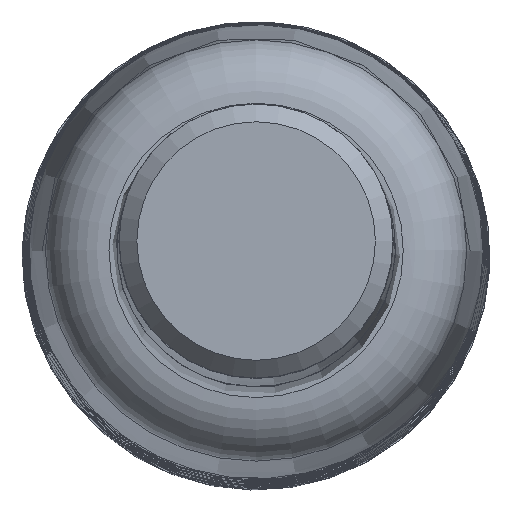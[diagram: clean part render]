
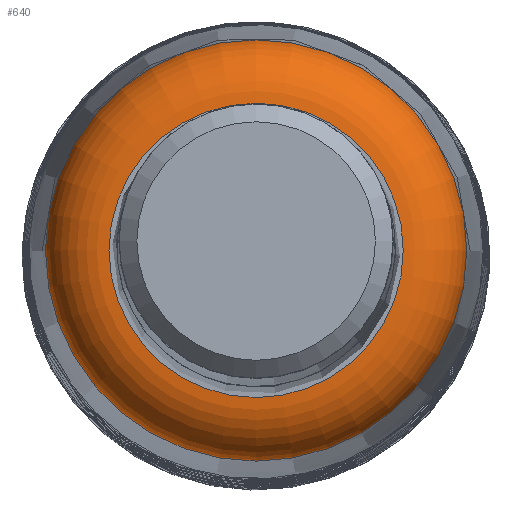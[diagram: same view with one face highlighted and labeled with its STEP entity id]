
A CAD part, top view. The second image highlights one B-rep face of the part: STEP entity #640.
In plain terms, the highlighted toroidal (fillet/blend) face has major radius 8.338 mm and minor radius 3.6 mm.
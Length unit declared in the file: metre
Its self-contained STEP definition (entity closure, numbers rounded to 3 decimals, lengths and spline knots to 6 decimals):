
#640=ADVANCED_FACE('',(#1492,#1493),#1494,.T.);
#1492=FACE_OUTER_BOUND('',#2652,.T.);
#1493=FACE_OUTER_BOUND('',#2653,.T.);
#1494=TOROIDAL_SURFACE('',#2654,0.008338,0.0036);
#2652=EDGE_LOOP('',(#4381));
#2653=EDGE_LOOP('',(#4382));
#2654=AXIS2_PLACEMENT_3D('',#4383,#4384,#4385);
#4381=ORIENTED_EDGE('',*,*,#5743,.F.);
#4382=ORIENTED_EDGE('',*,*,#6227,.F.);
#4383=CARTESIAN_POINT('',(0.,0.,0.1864));
#4384=DIRECTION('',(0.,0.,1.0));
#4385=DIRECTION('',(1.0,0.0,0.));
#5743=EDGE_CURVE('',#6738,#6738,#6739,.T.);
#6227=EDGE_CURVE('',#7544,#7544,#7545,.F.);
#6738=VERTEX_POINT('',#8180);
#6739=CIRCLE('',#8181,0.008338);
#7544=VERTEX_POINT('',#9542);
#7545=CIRCLE('',#9543,0.011937);
#8180=CARTESIAN_POINT('',(0.008338,0.,0.19));
#8181=AXIS2_PLACEMENT_3D('',#10447,#10448,#10449);
#9542=CARTESIAN_POINT('',(0.011937,0.,0.186488));
#9543=AXIS2_PLACEMENT_3D('',#11015,#11016,#11017);
#10447=CARTESIAN_POINT('',(0.,0.,0.19));
#10448=DIRECTION('',(0.,0.,1.0));
#10449=DIRECTION('',(1.0,0.0,0.));
#11015=CARTESIAN_POINT('',(0.0,0.0,0.186488));
#11016=DIRECTION('',(0.,0.,1.0));
#11017=DIRECTION('',(1.0,0.0,0.));
